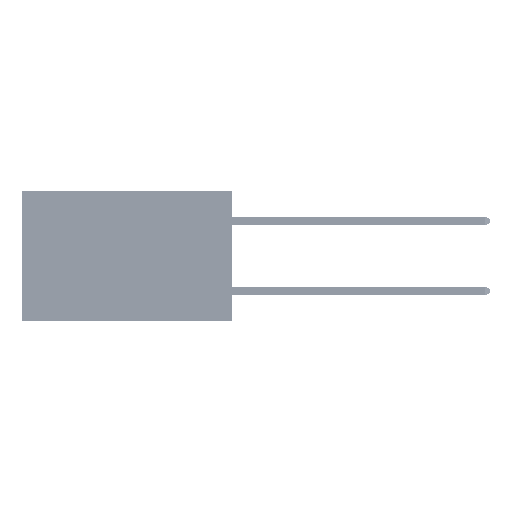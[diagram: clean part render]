
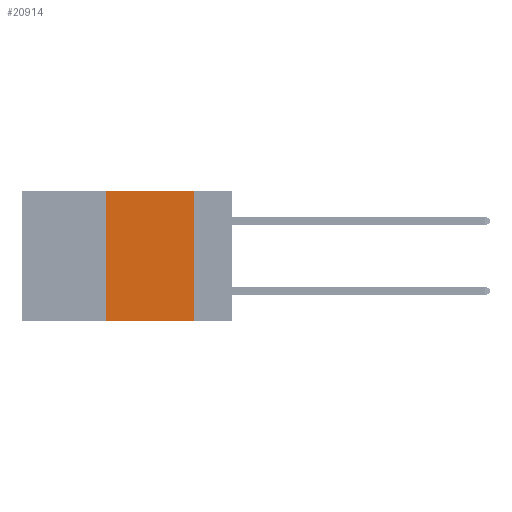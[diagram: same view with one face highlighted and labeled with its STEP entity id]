
A CAD part, left-side view. The second image highlights one B-rep face of the part: STEP entity #20914.
In plain terms, the highlighted planar face has unit normal (-1, 0, 0).
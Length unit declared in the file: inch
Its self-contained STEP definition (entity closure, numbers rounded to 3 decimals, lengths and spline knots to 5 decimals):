
#560 = ORIENTED_EDGE ( 'NONE', *, *, #3431, .F. ) ;
#2470 = LINE ( 'NONE', #19182, #46727 ) ;
#2991 = DIRECTION ( 'NONE',  ( 0., 0., -1. ) ) ;
#3431 = EDGE_CURVE ( 'NONE', #5177, #25475, #36306, .T. ) ;
#4880 = ORIENTED_EDGE ( 'NONE', *, *, #34829, .F. ) ;
#5177 = VERTEX_POINT ( 'NONE', #47210 ) ;
#5205 = EDGE_CURVE ( 'NONE', #35182, #25475, #38695, .T. ) ;
#5814 = CARTESIAN_POINT ( 'NONE',  ( 0., 0.6, -0.37 ) ) ;
#11605 = DIRECTION ( 'NONE',  ( 1., 0., 0. ) ) ;
#13342 = FACE_OUTER_BOUND ( 'NONE', #38767, .T. ) ;
#15497 = CARTESIAN_POINT ( 'NONE',  ( 0., 0.36, 0. ) ) ;
#17555 = VECTOR ( 'NONE', #40330, 39.37008 ) ;
#19182 = CARTESIAN_POINT ( 'NONE',  ( 0., 0.6, 0. ) ) ;
#20914 = ADVANCED_FACE ( 'NONE', ( #13342 ), #24010, .F. ) ;
#23767 = CARTESIAN_POINT ( 'NONE',  ( 0., 0.36, 0. ) ) ;
#24010 = PLANE ( 'NONE',  #41134 ) ;
#24809 = EDGE_CURVE ( 'NONE', #35182, #48676, #50575, .T. ) ;
#25274 = VECTOR ( 'NONE', #2991, 39.37008 ) ;
#25332 = CARTESIAN_POINT ( 'NONE',  ( 0., 0.36, -0.37 ) ) ;
#25475 = VERTEX_POINT ( 'NONE', #48374 ) ;
#28587 = ORIENTED_EDGE ( 'NONE', *, *, #5205, .T. ) ;
#34829 = EDGE_CURVE ( 'NONE', #48676, #5177, #2470, .T. ) ;
#35182 = VERTEX_POINT ( 'NONE', #25332 ) ;
#36306 = LINE ( 'NONE', #52724, #25274 ) ;
#36535 = CARTESIAN_POINT ( 'NONE',  ( 0., 0.6, 0. ) ) ;
#37398 = VECTOR ( 'NONE', #51501, 39.37008 ) ;
#38695 = LINE ( 'NONE', #5814, #37398 ) ;
#38767 = EDGE_LOOP ( 'NONE', ( #560, #4880, #49718, #28587 ) ) ;
#40330 = DIRECTION ( 'NONE',  ( 0., 0., 1. ) ) ;
#40669 = DIRECTION ( 'NONE',  ( 0., 0., -1. ) ) ;
#41134 = AXIS2_PLACEMENT_3D ( 'NONE', #36535, #11605, #40669 ) ;
#46727 = VECTOR ( 'NONE', #48137, 39.37008 ) ;
#47210 = CARTESIAN_POINT ( 'NONE',  ( 0., 0.11, 0. ) ) ;
#48137 = DIRECTION ( 'NONE',  ( 0., -1., 0. ) ) ;
#48374 = CARTESIAN_POINT ( 'NONE',  ( 0., 0.11, -0.37 ) ) ;
#48676 = VERTEX_POINT ( 'NONE', #23767 ) ;
#49718 = ORIENTED_EDGE ( 'NONE', *, *, #24809, .F. ) ;
#50575 = LINE ( 'NONE', #15497, #17555 ) ;
#51501 = DIRECTION ( 'NONE',  ( 0., -1., 0. ) ) ;
#52724 = CARTESIAN_POINT ( 'NONE',  ( 0., 0.11, 0. ) ) ;
